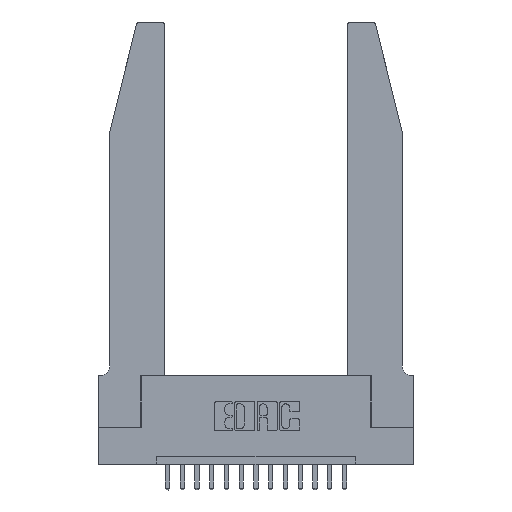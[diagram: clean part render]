
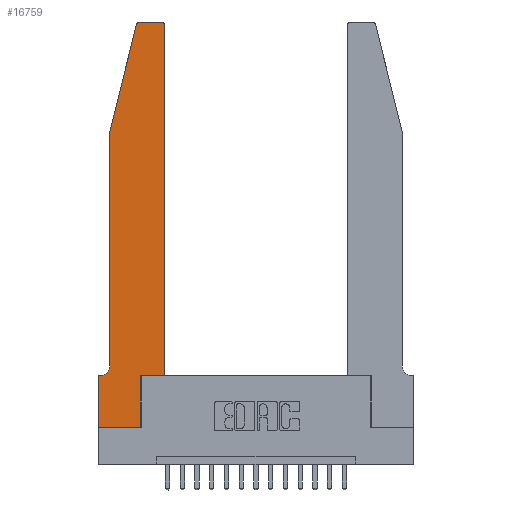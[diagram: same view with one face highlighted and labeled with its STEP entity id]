
A CAD part, top view. The second image highlights one B-rep face of the part: STEP entity #16759.
In plain terms, the highlighted planar face has unit normal (0, 0, 1).
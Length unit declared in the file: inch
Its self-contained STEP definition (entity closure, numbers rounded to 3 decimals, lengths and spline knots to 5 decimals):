
#51 = VECTOR ( 'NONE', #14033, 39.37008 ) ;
#213 = CARTESIAN_POINT ( 'NONE',  ( 0., 0.35, 0.37 ) ) ;
#315 = DIRECTION ( 'NONE',  ( 1., 0., 0. ) ) ;
#317 = CARTESIAN_POINT ( 'NONE',  ( 0., 0.35, 0.37 ) ) ;
#568 = CARTESIAN_POINT ( 'NONE',  ( 0.2865, 0., 0.37 ) ) ;
#690 = DIRECTION ( 'NONE',  ( -0.239, -0.971, 0. ) ) ;
#885 = VECTOR ( 'NONE', #315, 39.37008 ) ;
#1143 = CARTESIAN_POINT ( 'NONE',  ( 0.0755, 2., 0.37 ) ) ;
#1146 = ORIENTED_EDGE ( 'NONE', *, *, #16186, .T. ) ;
#1172 = CARTESIAN_POINT ( 'NONE',  ( 0.4205, 2.72, 0.37 ) ) ;
#1289 = ORIENTED_EDGE ( 'NONE', *, *, #4402, .T. ) ;
#1472 = ORIENTED_EDGE ( 'NONE', *, *, #4404, .T. ) ;
#1500 = AXIS2_PLACEMENT_3D ( 'NONE', #213, #8647, #10043 ) ;
#1648 = AXIS2_PLACEMENT_3D ( 'NONE', #15118, #5140, #2400 ) ;
#1698 = CARTESIAN_POINT ( 'NONE',  ( 0.4505, 0.35, 0.37 ) ) ;
#1869 = LINE ( 'NONE', #17712, #14163 ) ;
#2093 = EDGE_CURVE ( 'NONE', #3001, #4473, #9352, .T. ) ;
#2364 = CARTESIAN_POINT ( 'NONE',  ( 0., 0., 0.37 ) ) ;
#2400 = DIRECTION ( 'NONE',  ( 1., 0., 0. ) ) ;
#2471 = ORIENTED_EDGE ( 'NONE', *, *, #15853, .T. ) ;
#2511 = ORIENTED_EDGE ( 'NONE', *, *, #5744, .T. ) ;
#2725 = CARTESIAN_POINT ( 'NONE',  ( 0.0055, 0.35, 0.37 ) ) ;
#3001 = VERTEX_POINT ( 'NONE', #15075 ) ;
#3012 = DIRECTION ( 'NONE',  ( 0., 0., -1. ) ) ;
#3030 = CIRCLE ( 'NONE', #1648, 0.03 ) ;
#3108 = ORIENTED_EDGE ( 'NONE', *, *, #3210, .T. ) ;
#3180 = VECTOR ( 'NONE', #9368, 39.37008 ) ;
#3210 = EDGE_CURVE ( 'NONE', #4473, #13521, #3030, .T. ) ;
#3349 = AXIS2_PLACEMENT_3D ( 'NONE', #11557, #3012, #13004 ) ;
#3501 = DIRECTION ( 'NONE',  ( 0., -1., 0. ) ) ;
#4000 = LINE ( 'NONE', #1698, #885 ) ;
#4402 = EDGE_CURVE ( 'NONE', #16881, #3001, #10354, .T. ) ;
#4404 = EDGE_CURVE ( 'NONE', #6882, #8358, #9243, .T. ) ;
#4473 = VERTEX_POINT ( 'NONE', #11212 ) ;
#4994 = ORIENTED_EDGE ( 'NONE', *, *, #12821, .T. ) ;
#5082 = VECTOR ( 'NONE', #11746, 39.37008 ) ;
#5140 = DIRECTION ( 'NONE',  ( 0., 0., 1. ) ) ;
#5199 = EDGE_CURVE ( 'NONE', #12077, #16881, #1869, .T. ) ;
#5744 = EDGE_CURVE ( 'NONE', #9683, #6882, #17711, .T. ) ;
#5841 = LINE ( 'NONE', #14397, #6984 ) ;
#6798 = DIRECTION ( 'NONE',  ( 1., 0., 0. ) ) ;
#6882 = VERTEX_POINT ( 'NONE', #317 ) ;
#6984 = VECTOR ( 'NONE', #15916, 39.37008 ) ;
#7239 = CARTESIAN_POINT ( 'NONE',  ( 0.2605, 2.75, 0.37 ) ) ;
#7420 = VERTEX_POINT ( 'NONE', #1143 ) ;
#8358 = VERTEX_POINT ( 'NONE', #8526 ) ;
#8526 = CARTESIAN_POINT ( 'NONE',  ( 0., 0., 0.37 ) ) ;
#8647 = DIRECTION ( 'NONE',  ( 0., 0., 1. ) ) ;
#9130 = EDGE_CURVE ( 'NONE', #13521, #7420, #9922, .T. ) ;
#9243 = LINE ( 'NONE', #12524, #51 ) ;
#9352 = LINE ( 'NONE', #7239, #5082 ) ;
#9368 = DIRECTION ( 'NONE',  ( -1., 0., 0. ) ) ;
#9374 = CIRCLE ( 'NONE', #3349, 0.07 ) ;
#9476 = AXIS2_PLACEMENT_3D ( 'NONE', #1172, #14160, #11086 ) ;
#9683 = VERTEX_POINT ( 'NONE', #2725 ) ;
#9820 = EDGE_CURVE ( 'NONE', #13892, #11181, #5841, .T. ) ;
#9922 = LINE ( 'NONE', #10505, #17978 ) ;
#10043 = DIRECTION ( 'NONE',  ( 1., 0., 0. ) ) ;
#10263 = LINE ( 'NONE', #13393, #16569 ) ;
#10354 = CIRCLE ( 'NONE', #9476, 0.03 ) ;
#10505 = CARTESIAN_POINT ( 'NONE',  ( 0.0755, 2., 0.37 ) ) ;
#11086 = DIRECTION ( 'NONE',  ( 1., 0., 0. ) ) ;
#11181 = VERTEX_POINT ( 'NONE', #14845 ) ;
#11212 = CARTESIAN_POINT ( 'NONE',  ( 0.284, 2.75, 0.37 ) ) ;
#11417 = EDGE_LOOP ( 'NONE', ( #17080, #3108, #16696, #4994, #1146, #2511, #1472, #15908, #15714, #2471, #16582, #1289 ) ) ;
#11557 = CARTESIAN_POINT ( 'NONE',  ( 0.0055, 0.42, 0.37 ) ) ;
#11746 = DIRECTION ( 'NONE',  ( -1., 0., 0. ) ) ;
#12077 = VERTEX_POINT ( 'NONE', #18426 ) ;
#12524 = CARTESIAN_POINT ( 'NONE',  ( 0., 0., 0.37 ) ) ;
#12821 = EDGE_CURVE ( 'NONE', #7420, #12993, #10263, .T. ) ;
#12993 = VERTEX_POINT ( 'NONE', #17018 ) ;
#13004 = DIRECTION ( 'NONE',  ( -1., 0., 0. ) ) ;
#13005 = EDGE_CURVE ( 'NONE', #8358, #13892, #14993, .T. ) ;
#13393 = CARTESIAN_POINT ( 'NONE',  ( 0.0755, 2., 0.37 ) ) ;
#13521 = VERTEX_POINT ( 'NONE', #13840 ) ;
#13840 = CARTESIAN_POINT ( 'NONE',  ( 0.25487, 2.72718, 0.37 ) ) ;
#13892 = VERTEX_POINT ( 'NONE', #568 ) ;
#14033 = DIRECTION ( 'NONE',  ( 0., -1., 0. ) ) ;
#14160 = DIRECTION ( 'NONE',  ( 0., 0., 1. ) ) ;
#14163 = VECTOR ( 'NONE', #17845, 39.37008 ) ;
#14397 = CARTESIAN_POINT ( 'NONE',  ( 0.2865, 0.35, 0.37 ) ) ;
#14602 = CARTESIAN_POINT ( 'NONE',  ( 0.4505, 2.72, 0.37 ) ) ;
#14845 = CARTESIAN_POINT ( 'NONE',  ( 0.2865, 0.35, 0.37 ) ) ;
#14993 = LINE ( 'NONE', #2364, #17400 ) ;
#15075 = CARTESIAN_POINT ( 'NONE',  ( 0.4205, 2.75, 0.37 ) ) ;
#15118 = CARTESIAN_POINT ( 'NONE',  ( 0.284, 2.72, 0.37 ) ) ;
#15714 = ORIENTED_EDGE ( 'NONE', *, *, #9820, .T. ) ;
#15853 = EDGE_CURVE ( 'NONE', #11181, #12077, #4000, .T. ) ;
#15908 = ORIENTED_EDGE ( 'NONE', *, *, #13005, .T. ) ;
#15916 = DIRECTION ( 'NONE',  ( 0., 1., 0. ) ) ;
#16186 = EDGE_CURVE ( 'NONE', #12993, #9683, #9374, .T. ) ;
#16569 = VECTOR ( 'NONE', #3501, 39.37008 ) ;
#16575 = CARTESIAN_POINT ( 'NONE',  ( 0.0755, 0.35, 0.37 ) ) ;
#16582 = ORIENTED_EDGE ( 'NONE', *, *, #5199, .T. ) ;
#16696 = ORIENTED_EDGE ( 'NONE', *, *, #9130, .T. ) ;
#16759 = ADVANCED_FACE ( 'NONE', ( #17403 ), #17309, .T. ) ;
#16881 = VERTEX_POINT ( 'NONE', #14602 ) ;
#17018 = CARTESIAN_POINT ( 'NONE',  ( 0.0755, 0.42, 0.37 ) ) ;
#17080 = ORIENTED_EDGE ( 'NONE', *, *, #2093, .T. ) ;
#17309 = PLANE ( 'NONE',  #1500 ) ;
#17400 = VECTOR ( 'NONE', #6798, 39.37008 ) ;
#17403 = FACE_OUTER_BOUND ( 'NONE', #11417, .T. ) ;
#17711 = LINE ( 'NONE', #16575, #3180 ) ;
#17712 = CARTESIAN_POINT ( 'NONE',  ( 0.4505, 0.35, 0.37 ) ) ;
#17845 = DIRECTION ( 'NONE',  ( 0., 1., 0. ) ) ;
#17978 = VECTOR ( 'NONE', #690, 39.37008 ) ;
#18426 = CARTESIAN_POINT ( 'NONE',  ( 0.4505, 0.35, 0.37 ) ) ;
